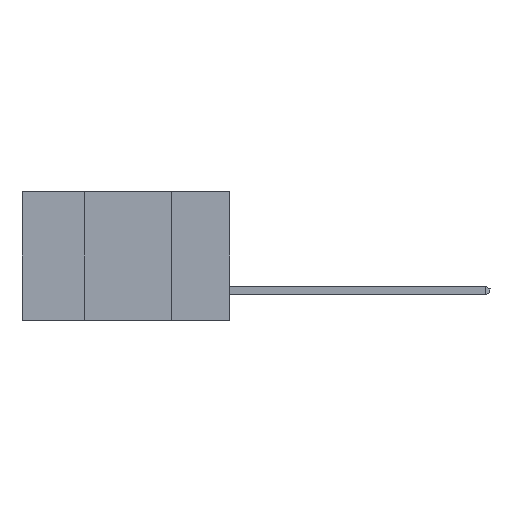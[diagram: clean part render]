
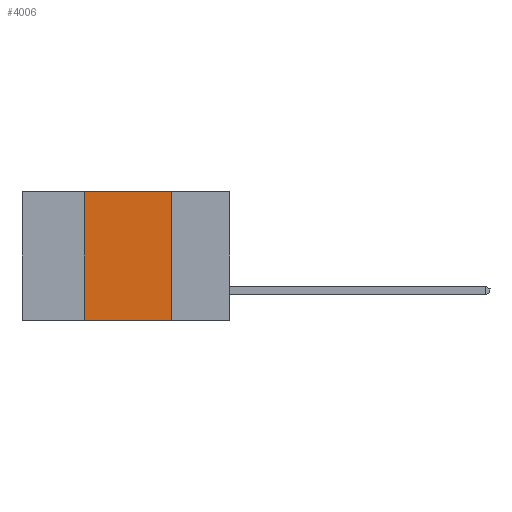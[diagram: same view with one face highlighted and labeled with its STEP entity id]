
A CAD part, left-side view. The second image highlights one B-rep face of the part: STEP entity #4006.
In plain terms, the highlighted planar face has unit normal (-1, 0, 0).
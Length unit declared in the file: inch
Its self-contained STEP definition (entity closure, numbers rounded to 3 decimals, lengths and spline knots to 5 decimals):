
#862 = VECTOR ( 'NONE', #1601, 39.37008 ) ;
#1298 = VECTOR ( 'NONE', #15759, 39.37008 ) ;
#1497 = CARTESIAN_POINT ( 'NONE',  ( 0., 0.17, -0.37 ) ) ;
#1601 = DIRECTION ( 'NONE',  ( 0., 0., -1. ) ) ;
#2002 = CARTESIAN_POINT ( 'NONE',  ( 0., 0.17, 0. ) ) ;
#2482 = VECTOR ( 'NONE', #8893, 39.37008 ) ;
#4006 = ADVANCED_FACE ( 'NONE', ( #15335 ), #11979, .F. ) ;
#4188 = EDGE_CURVE ( 'NONE', #13381, #7926, #4741, .T. ) ;
#4689 = CARTESIAN_POINT ( 'NONE',  ( 0., 0.42, -0.37 ) ) ;
#4741 = LINE ( 'NONE', #17449, #1298 ) ;
#5214 = ORIENTED_EDGE ( 'NONE', *, *, #20659, .T. ) ;
#6372 = LINE ( 'NONE', #4689, #17964 ) ;
#6738 = ORIENTED_EDGE ( 'NONE', *, *, #7840, .F. ) ;
#7166 = DIRECTION ( 'NONE',  ( 0., 0., -1. ) ) ;
#7265 = DIRECTION ( 'NONE',  ( 1., 0., 0. ) ) ;
#7449 = EDGE_CURVE ( 'NONE', #18428, #13381, #6372, .T. ) ;
#7840 = EDGE_CURVE ( 'NONE', #7926, #17607, #15987, .T. ) ;
#7926 = VERTEX_POINT ( 'NONE', #2002 ) ;
#8893 = DIRECTION ( 'NONE',  ( 0., -1., 0. ) ) ;
#10197 = CARTESIAN_POINT ( 'NONE',  ( 0., 0.42, -0.37 ) ) ;
#10671 = CARTESIAN_POINT ( 'NONE',  ( 0., 0.6, -0.37 ) ) ;
#11979 = PLANE ( 'NONE',  #14616 ) ;
#12109 = ORIENTED_EDGE ( 'NONE', *, *, #4188, .F. ) ;
#13381 = VERTEX_POINT ( 'NONE', #17408 ) ;
#13602 = ORIENTED_EDGE ( 'NONE', *, *, #7449, .F. ) ;
#14475 = EDGE_LOOP ( 'NONE', ( #6738, #12109, #13602, #5214 ) ) ;
#14518 = CARTESIAN_POINT ( 'NONE',  ( 0., 0.17, -0.37 ) ) ;
#14616 = AXIS2_PLACEMENT_3D ( 'NONE', #20066, #7265, #7166 ) ;
#15335 = FACE_OUTER_BOUND ( 'NONE', #14475, .T. ) ;
#15759 = DIRECTION ( 'NONE',  ( 0., -1., 0. ) ) ;
#15914 = DIRECTION ( 'NONE',  ( 0., 0., 1. ) ) ;
#15987 = LINE ( 'NONE', #14518, #862 ) ;
#16972 = LINE ( 'NONE', #10671, #2482 ) ;
#17408 = CARTESIAN_POINT ( 'NONE',  ( 0., 0.42, 0. ) ) ;
#17449 = CARTESIAN_POINT ( 'NONE',  ( 0., 0.6, 0. ) ) ;
#17607 = VERTEX_POINT ( 'NONE', #1497 ) ;
#17964 = VECTOR ( 'NONE', #15914, 39.37008 ) ;
#18428 = VERTEX_POINT ( 'NONE', #10197 ) ;
#20066 = CARTESIAN_POINT ( 'NONE',  ( 0., 0.6, 0. ) ) ;
#20659 = EDGE_CURVE ( 'NONE', #18428, #17607, #16972, .T. ) ;
